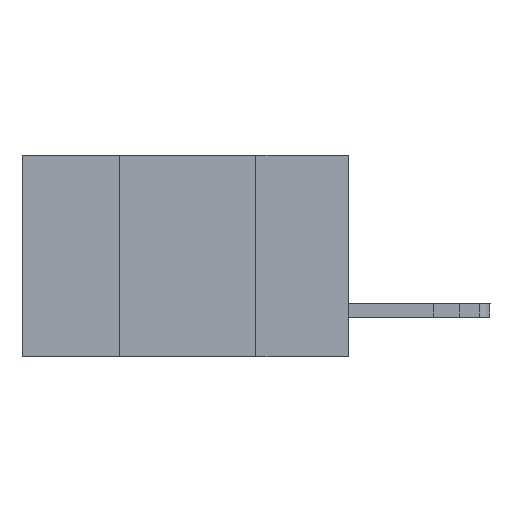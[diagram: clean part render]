
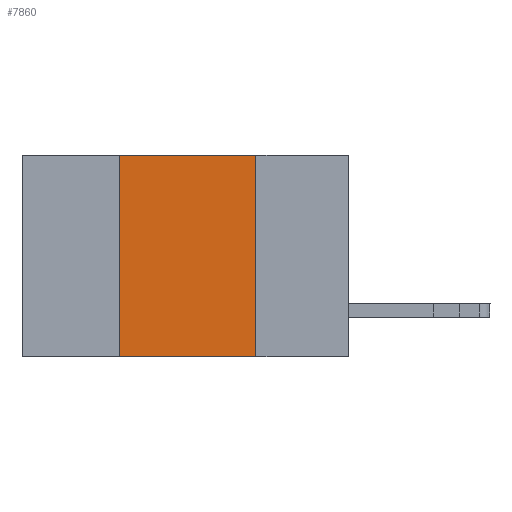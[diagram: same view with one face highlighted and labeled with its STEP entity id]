
A CAD part, left-side view. The second image highlights one B-rep face of the part: STEP entity #7860.
In plain terms, the highlighted planar face has unit normal (-1, 0, 0).
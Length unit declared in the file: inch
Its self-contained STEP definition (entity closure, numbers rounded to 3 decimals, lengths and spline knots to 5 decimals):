
#202 = CARTESIAN_POINT ( 'NONE',  ( 0., 0.6, 0. ) ) ;
#676 = VERTEX_POINT ( 'NONE', #4489 ) ;
#1956 = CARTESIAN_POINT ( 'NONE',  ( 0., 0.17, -0.37 ) ) ;
#2101 = DIRECTION ( 'NONE',  ( 0., 0., -1. ) ) ;
#4148 = LINE ( 'NONE', #10618, #12158 ) ;
#4477 = CARTESIAN_POINT ( 'NONE',  ( 0., 0.17, 0. ) ) ;
#4489 = CARTESIAN_POINT ( 'NONE',  ( 0., 0.42, 0. ) ) ;
#4508 = DIRECTION ( 'NONE',  ( 1., 0., 0. ) ) ;
#4625 = CARTESIAN_POINT ( 'NONE',  ( 0., 0.17, -0.37 ) ) ;
#5137 = ORIENTED_EDGE ( 'NONE', *, *, #8490, .F. ) ;
#5240 = LINE ( 'NONE', #10848, #10748 ) ;
#5354 = VECTOR ( 'NONE', #13995, 39.37008 ) ;
#5362 = ORIENTED_EDGE ( 'NONE', *, *, #14163, .T. ) ;
#5659 = PLANE ( 'NONE',  #13093 ) ;
#6184 = LINE ( 'NONE', #10563, #5354 ) ;
#6355 = EDGE_CURVE ( 'NONE', #676, #13434, #4148, .T. ) ;
#6400 = DIRECTION ( 'NONE',  ( 0., 0., 1. ) ) ;
#7643 = VECTOR ( 'NONE', #2101, 39.37008 ) ;
#7860 = ADVANCED_FACE ( 'NONE', ( #9967 ), #5659, .F. ) ;
#8490 = EDGE_CURVE ( 'NONE', #13434, #11156, #10588, .T. ) ;
#8897 = DIRECTION ( 'NONE',  ( 0., 0., -1. ) ) ;
#8976 = EDGE_LOOP ( 'NONE', ( #5137, #9365, #11045, #5362 ) ) ;
#9365 = ORIENTED_EDGE ( 'NONE', *, *, #6355, .F. ) ;
#9777 = CARTESIAN_POINT ( 'NONE',  ( 0., 0.42, -0.37 ) ) ;
#9967 = FACE_OUTER_BOUND ( 'NONE', #8976, .T. ) ;
#10024 = EDGE_CURVE ( 'NONE', #12697, #676, #5240, .T. ) ;
#10563 = CARTESIAN_POINT ( 'NONE',  ( 0., 0.6, -0.37 ) ) ;
#10588 = LINE ( 'NONE', #1956, #7643 ) ;
#10618 = CARTESIAN_POINT ( 'NONE',  ( 0., 0.6, 0. ) ) ;
#10748 = VECTOR ( 'NONE', #6400, 39.37008 ) ;
#10848 = CARTESIAN_POINT ( 'NONE',  ( 0., 0.42, -0.37 ) ) ;
#11045 = ORIENTED_EDGE ( 'NONE', *, *, #10024, .F. ) ;
#11156 = VERTEX_POINT ( 'NONE', #4625 ) ;
#12158 = VECTOR ( 'NONE', #13983, 39.37008 ) ;
#12697 = VERTEX_POINT ( 'NONE', #9777 ) ;
#13093 = AXIS2_PLACEMENT_3D ( 'NONE', #202, #4508, #8897 ) ;
#13434 = VERTEX_POINT ( 'NONE', #4477 ) ;
#13983 = DIRECTION ( 'NONE',  ( 0., -1., 0. ) ) ;
#13995 = DIRECTION ( 'NONE',  ( 0., -1., 0. ) ) ;
#14163 = EDGE_CURVE ( 'NONE', #12697, #11156, #6184, .T. ) ;
